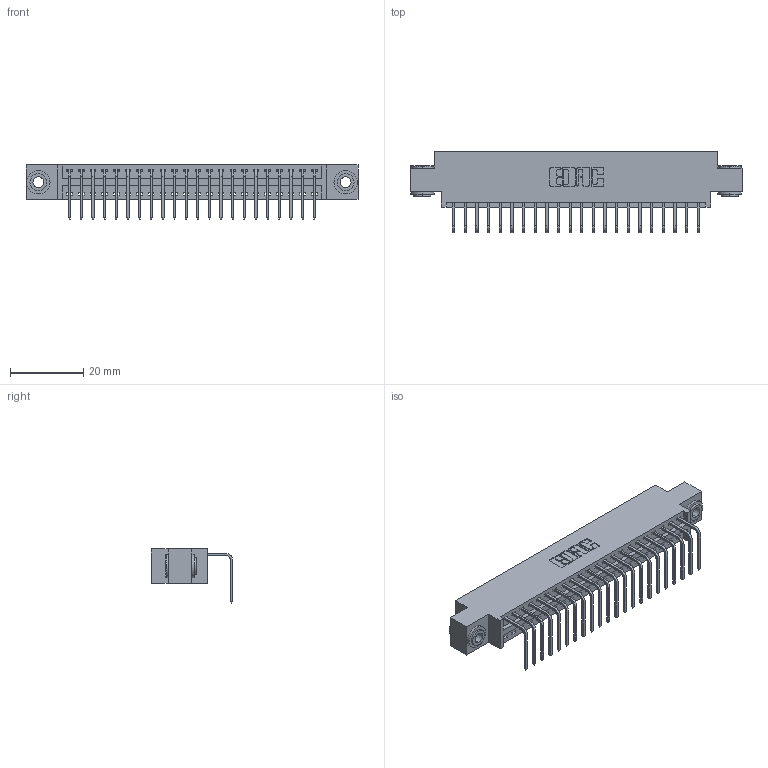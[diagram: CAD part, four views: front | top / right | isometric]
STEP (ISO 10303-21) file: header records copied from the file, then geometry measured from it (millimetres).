
FILE_DESCRIPTION (( 'STEP AP203' ), '1' );
FILE_NAME ('346-022-558-603.STEP', '2022-05-05T20:09:01', ( '' ), ( '' ), 'SwSTEP 2.0', 'SolidWorks 2020', '' );
FILE_SCHEMA (( 'CONFIG_CONTROL_DESIGN' ));
Length unit declared in the file: inch
Products named in the file (4): 345-250-002_345-250-002-102; 346 Part_0.170 Offset - 0.156 Dia-TH; 346-022-558-603; 345-292-001_558 Tail - 2
Assembly tree (25 placements, depth 2):
  346-022-558-603
    346 Part_0.170 Offset - 0.156 Dia-TH
    345-292-001_558 Tail - 2  x22
    345-250-002_345-250-002-102  x2
Bounding box: 90.42 x 22.16 x 14.73 mm (x, y, z)
Volume: 8437.8 mm3; surface area: 11179.4 mm2
Topology: 25 solids, 25 shells, 1498 faces, 4457 edges, 2938 vertices
Faces by surface type: plane 1028, cylinder 462, cone 8
Entity records: 17628 total; most frequent: CARTESIAN_POINT 3011, ORIENTED_EDGE 2958, DIRECTION 2709, EDGE_CURVE 1479, VECTOR 1235, LINE 1235, VERTEX_POINT 982, AXIS2_PLACEMENT_3D 737
